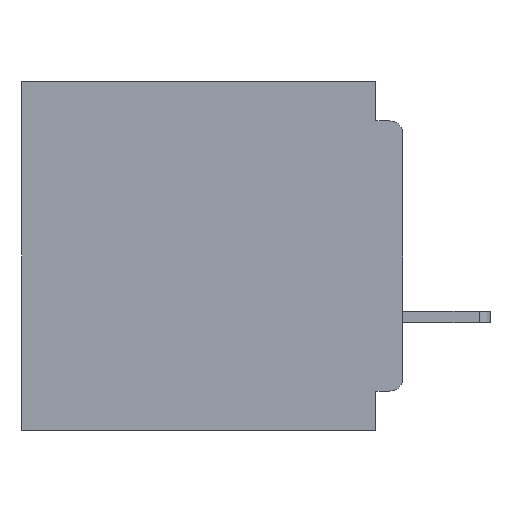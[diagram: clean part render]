
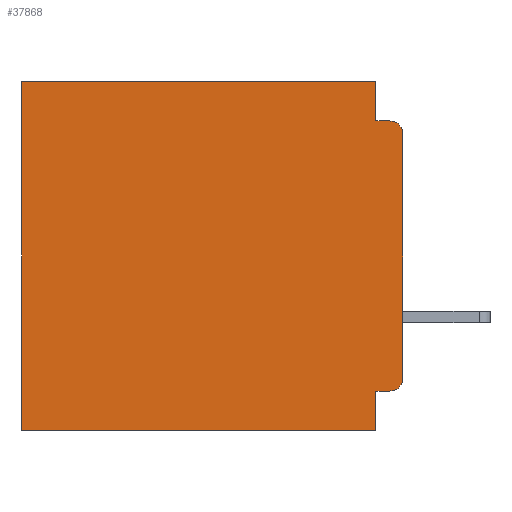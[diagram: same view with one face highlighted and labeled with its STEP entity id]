
A CAD part, left-side view. The second image highlights one B-rep face of the part: STEP entity #37868.
In plain terms, the highlighted planar face has unit normal (-1, 0, 0).
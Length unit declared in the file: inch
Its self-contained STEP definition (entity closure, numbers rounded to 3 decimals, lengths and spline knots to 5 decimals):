
#544 = CARTESIAN_POINT ( 'NONE',  ( 0.3, 0.015, -0.06 ) ) ;
#560 = VECTOR ( 'NONE', #51040, 39.37008 ) ;
#656 = ORIENTED_EDGE ( 'NONE', *, *, #37203, .T. ) ;
#711 = EDGE_LOOP ( 'NONE', ( #30445, #656, #51468, #45130, #37530, #32426, #10360, #7404, #45124, #6979 ) ) ;
#987 = CIRCLE ( 'NONE', #20650, 0.015 ) ;
#1056 = EDGE_CURVE ( 'NONE', #26230, #56636, #52373, .T. ) ;
#2115 = EDGE_CURVE ( 'NONE', #12351, #49631, #42087, .T. ) ;
#3090 = DIRECTION ( 'NONE',  ( 0., 1., 0. ) ) ;
#3763 = CARTESIAN_POINT ( 'NONE',  ( 0.3, 0.031, -0.355 ) ) ;
#5044 = EDGE_CURVE ( 'NONE', #24147, #7444, #45745, .T. ) ;
#5313 = DIRECTION ( 'NONE',  ( 0., 0., -1. ) ) ;
#6000 = AXIS2_PLACEMENT_3D ( 'NONE', #25087, #57764, #29798 ) ;
#6979 = ORIENTED_EDGE ( 'NONE', *, *, #32790, .T. ) ;
#7089 = CARTESIAN_POINT ( 'NONE',  ( 0.3, 0.437, 0. ) ) ;
#7404 = ORIENTED_EDGE ( 'NONE', *, *, #1056, .F. ) ;
#7444 = VERTEX_POINT ( 'NONE', #47872 ) ;
#7806 = VECTOR ( 'NONE', #27573, 39.37008 ) ;
#9941 = CARTESIAN_POINT ( 'NONE',  ( 0.3, 0., -0.4 ) ) ;
#10360 = ORIENTED_EDGE ( 'NONE', *, *, #35998, .F. ) ;
#12351 = VERTEX_POINT ( 'NONE', #30687 ) ;
#13630 = EDGE_CURVE ( 'NONE', #26916, #59182, #15026, .T. ) ;
#14629 = DIRECTION ( 'NONE',  ( 1., 0., 0. ) ) ;
#15026 = LINE ( 'NONE', #19393, #40003 ) ;
#15969 = LINE ( 'NONE', #46339, #560 ) ;
#16255 = EDGE_CURVE ( 'NONE', #22175, #26916, #54349, .T. ) ;
#16759 = CARTESIAN_POINT ( 'NONE',  ( 0.3, 0.031, -0.045 ) ) ;
#19393 = CARTESIAN_POINT ( 'NONE',  ( 0.3, 0., -0.045 ) ) ;
#20142 = CARTESIAN_POINT ( 'NONE',  ( 0.3, 0., -0.34 ) ) ;
#20650 = AXIS2_PLACEMENT_3D ( 'NONE', #544, #33376, #5313 ) ;
#22175 = VERTEX_POINT ( 'NONE', #51228 ) ;
#24147 = VERTEX_POINT ( 'NONE', #7089 ) ;
#25087 = CARTESIAN_POINT ( 'NONE',  ( 0.3, 0.015, -0.34 ) ) ;
#26230 = VERTEX_POINT ( 'NONE', #3763 ) ;
#26916 = VERTEX_POINT ( 'NONE', #16759 ) ;
#27573 = DIRECTION ( 'NONE',  ( 0., 1., 0. ) ) ;
#28870 = DIRECTION ( 'NONE',  ( 0., -1., 0. ) ) ;
#29798 = DIRECTION ( 'NONE',  ( 0., 0., -1. ) ) ;
#30445 = ORIENTED_EDGE ( 'NONE', *, *, #2115, .F. ) ;
#30687 = CARTESIAN_POINT ( 'NONE',  ( 0.3, 0., -0.06 ) ) ;
#30922 = AXIS2_PLACEMENT_3D ( 'NONE', #9941, #14629, #47347 ) ;
#31673 = VECTOR ( 'NONE', #3090, 39.37008 ) ;
#32426 = ORIENTED_EDGE ( 'NONE', *, *, #5044, .T. ) ;
#32790 = EDGE_CURVE ( 'NONE', #56102, #49631, #55690, .T. ) ;
#33376 = DIRECTION ( 'NONE',  ( -1., 0., 0. ) ) ;
#35863 = CARTESIAN_POINT ( 'NONE',  ( 0.3, 0.031, -0.4 ) ) ;
#35998 = EDGE_CURVE ( 'NONE', #56636, #7444, #45119, .T. ) ;
#36792 = CARTESIAN_POINT ( 'NONE',  ( 0.3, 0., -0.4 ) ) ;
#37203 = EDGE_CURVE ( 'NONE', #12351, #59182, #987, .T. ) ;
#37530 = ORIENTED_EDGE ( 'NONE', *, *, #58964, .T. ) ;
#37610 = FACE_OUTER_BOUND ( 'NONE', #711, .T. ) ;
#37868 = ADVANCED_FACE ( 'NONE', ( #37610 ), #38001, .F. ) ;
#38001 = PLANE ( 'NONE',  #30922 ) ;
#38420 = EDGE_CURVE ( 'NONE', #56102, #26230, #42643, .T. ) ;
#39742 = DIRECTION ( 'NONE',  ( 0., 0., -1. ) ) ;
#40003 = VECTOR ( 'NONE', #28870, 39.37008 ) ;
#40047 = VECTOR ( 'NONE', #46869, 39.37008 ) ;
#40638 = VECTOR ( 'NONE', #39742, 39.37008 ) ;
#42087 = LINE ( 'NONE', #56303, #40638 ) ;
#42643 = LINE ( 'NONE', #45264, #31673 ) ;
#43528 = CARTESIAN_POINT ( 'NONE',  ( 0.3, 0.437, -0.4 ) ) ;
#45119 = LINE ( 'NONE', #36792, #7806 ) ;
#45124 = ORIENTED_EDGE ( 'NONE', *, *, #38420, .F. ) ;
#45130 = ORIENTED_EDGE ( 'NONE', *, *, #16255, .F. ) ;
#45264 = CARTESIAN_POINT ( 'NONE',  ( 0.3, 0., -0.355 ) ) ;
#45745 = LINE ( 'NONE', #43528, #58143 ) ;
#46328 = VECTOR ( 'NONE', #51833, 39.37008 ) ;
#46339 = CARTESIAN_POINT ( 'NONE',  ( 0.3, 0., 0. ) ) ;
#46869 = DIRECTION ( 'NONE',  ( 0., 0., -1. ) ) ;
#47347 = DIRECTION ( 'NONE',  ( 0., 0., -1. ) ) ;
#47872 = CARTESIAN_POINT ( 'NONE',  ( 0.3, 0.437, -0.4 ) ) ;
#49631 = VERTEX_POINT ( 'NONE', #20142 ) ;
#51040 = DIRECTION ( 'NONE',  ( 0., 1., 0. ) ) ;
#51228 = CARTESIAN_POINT ( 'NONE',  ( 0.3, 0.031, 0. ) ) ;
#51468 = ORIENTED_EDGE ( 'NONE', *, *, #13630, .F. ) ;
#51833 = DIRECTION ( 'NONE',  ( 0., 0., -1. ) ) ;
#52373 = LINE ( 'NONE', #58674, #40047 ) ;
#54349 = LINE ( 'NONE', #56507, #46328 ) ;
#54456 = CARTESIAN_POINT ( 'NONE',  ( 0.3, 0.015, -0.355 ) ) ;
#55690 = CIRCLE ( 'NONE', #6000, 0.015 ) ;
#56102 = VERTEX_POINT ( 'NONE', #54456 ) ;
#56303 = CARTESIAN_POINT ( 'NONE',  ( 0.3, 0., -0.4 ) ) ;
#56507 = CARTESIAN_POINT ( 'NONE',  ( 0.3, 0.031, 0. ) ) ;
#56636 = VERTEX_POINT ( 'NONE', #35863 ) ;
#57517 = CARTESIAN_POINT ( 'NONE',  ( 0.3, 0.015, -0.045 ) ) ;
#57572 = DIRECTION ( 'NONE',  ( 0., 0., -1. ) ) ;
#57764 = DIRECTION ( 'NONE',  ( -1., 0., 0. ) ) ;
#58143 = VECTOR ( 'NONE', #57572, 39.37008 ) ;
#58674 = CARTESIAN_POINT ( 'NONE',  ( 0.3, 0.031, -0.4 ) ) ;
#58964 = EDGE_CURVE ( 'NONE', #22175, #24147, #15969, .T. ) ;
#59182 = VERTEX_POINT ( 'NONE', #57517 ) ;
